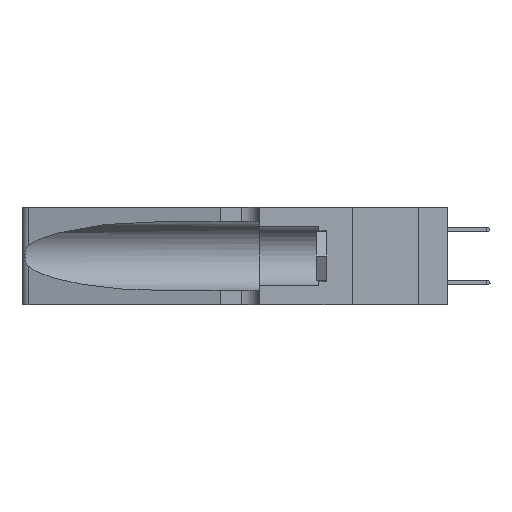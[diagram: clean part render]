
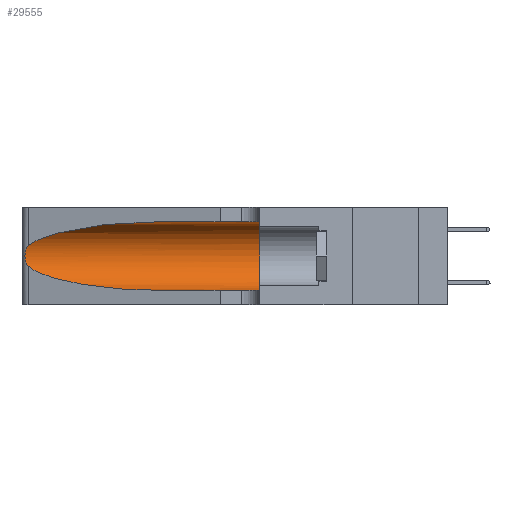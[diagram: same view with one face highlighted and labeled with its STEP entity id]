
A CAD part, left-side view. The second image highlights one B-rep face of the part: STEP entity #29555.
In plain terms, the highlighted cylindrical face has radius 3.308 mm (diameter 6.617 mm), a partial arc.
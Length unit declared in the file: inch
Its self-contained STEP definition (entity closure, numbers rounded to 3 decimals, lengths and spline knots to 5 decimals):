
#559 = CARTESIAN_POINT ( 'NONE',  ( 0.25787, 1.23484, 0.2124 ) ) ;
#2589 = CARTESIAN_POINT ( 'NONE',  ( 0.1305, 1.61858, 0.31525 ) ) ;
#2874 = ORIENTED_EDGE ( 'NONE', *, *, #18999, .T. ) ;
#3342 = CARTESIAN_POINT ( 'NONE',  ( 0.25856, 1.23593, 0.16098 ) ) ;
#3909 = CARTESIAN_POINT ( 'NONE',  ( 0.2373, 1.15595, 0.08982 ) ) ;
#4767 = ORIENTED_EDGE ( 'NONE', *, *, #8460, .T. ) ;
#4865 = DIRECTION ( 'NONE',  ( 0., 1., 0. ) ) ;
#4882 =( BOUNDED_CURVE ( )  B_SPLINE_CURVE ( 3, ( #11950, #3909, #14658, #31008 ),
 .UNSPECIFIED., .F., .F. ) 
 B_SPLINE_CURVE_WITH_KNOTS ( ( 4, 4 ),
 ( 3.44316, 4.71239 ),
 .UNSPECIFIED. ) 
 CURVE ( )  GEOMETRIC_REPRESENTATION_ITEM ( )  RATIONAL_B_SPLINE_CURVE ( ( 1., 0.87, 0.87, 1. ) ) 
 REPRESENTATION_ITEM ( '' )  );
#6047 = CARTESIAN_POINT ( 'NONE',  ( 0.25555, 1.22993, 0.14849 ) ) ;
#6652 = CARTESIAN_POINT ( 'NONE',  ( 0.1305, 1.61858, 0.185 ) ) ;
#6842 = CARTESIAN_POINT ( 'NONE',  ( 0.1305, 0.35, 0.31525 ) ) ;
#7187 = CARTESIAN_POINT ( 'NONE',  ( 0.1305, 0.72297, 0.31525 ) ) ;
#7802 = CARTESIAN_POINT ( 'NONE',  ( 0.1305, 0.72297, 0.31525 ) ) ;
#8460 = EDGE_CURVE ( 'NONE', #31767, #15767, #31958, .T. ) ;
#8649 = CARTESIAN_POINT ( 'NONE',  ( 0.26075, 1.23896, 0.19203 ) ) ;
#10161 = CARTESIAN_POINT ( 'NONE',  ( 0.18966, 0.96281, 0.31525 ) ) ;
#11276 = CARTESIAN_POINT ( 'NONE',  ( 0.25555, 1.22994, 0.2215 ) ) ;
#11371 = ORIENTED_EDGE ( 'NONE', *, *, #24735, .F. ) ;
#11396 = CARTESIAN_POINT ( 'NONE',  ( 0.26075, 1.23896, 0.178 ) ) ;
#11507 = CARTESIAN_POINT ( 'NONE',  ( 0.25487, 1.22718, 0.14631 ) ) ;
#11719 = LINE ( 'NONE', #24956, #23043 ) ;
#11950 = CARTESIAN_POINT ( 'NONE',  ( 0.25487, 1.22718, 0.14631 ) ) ;
#12204 = CARTESIAN_POINT ( 'NONE',  ( 0.25487, 1.22718, 0.14631 ) ) ;
#14658 = CARTESIAN_POINT ( 'NONE',  ( 0.18966, 0.96281, 0.05475 ) ) ;
#15136 = EDGE_CURVE ( 'NONE', #31767, #25947, #27100, .T. ) ;
#15450 = CARTESIAN_POINT ( 'NONE',  ( 0.2373, 1.15595, 0.28018 ) ) ;
#15749 = EDGE_CURVE ( 'NONE', #26336, #24824, #4882, .T. ) ;
#15767 = VERTEX_POINT ( 'NONE', #28085 ) ;
#16781 = CARTESIAN_POINT ( 'NONE',  ( 0.25789, 1.23486, 0.15765 ) ) ;
#17059 = CIRCLE ( 'NONE', #29937, 0.13025 ) ;
#18683 = FACE_OUTER_BOUND ( 'NONE', #33144, .T. ) ;
#18999 = EDGE_CURVE ( 'NONE', #15767, #26336, #33882, .T. ) ;
#19575 = DIRECTION ( 'NONE',  ( 0., -1., 0. ) ) ;
#20334 = CYLINDRICAL_SURFACE ( 'NONE', #22836, 0.13025 ) ;
#20994 = CARTESIAN_POINT ( 'NONE',  ( 0.1305, 0.35, 0.185 ) ) ;
#21076 = DIRECTION ( 'NONE',  ( 0., -1., 0. ) ) ;
#21408 = CARTESIAN_POINT ( 'NONE',  ( 0.1305, 0.72297, 0.05475 ) ) ;
#22061 = CARTESIAN_POINT ( 'NONE',  ( 0.25854, 1.2359, 0.20912 ) ) ;
#22167 = CARTESIAN_POINT ( 'NONE',  ( 0.25639, 1.23186, 0.15144 ) ) ;
#22613 = CARTESIAN_POINT ( 'NONE',  ( 0.1305, 0.35, 0.05475 ) ) ;
#22836 = AXIS2_PLACEMENT_3D ( 'NONE', #6652, #24653, #30121 ) ;
#23043 = VECTOR ( 'NONE', #19575, 39.37008 ) ;
#23219 = ORIENTED_EDGE ( 'NONE', *, *, #15749, .T. ) ;
#23647 = EDGE_CURVE ( 'NONE', #24824, #34590, #11719, .T. ) ;
#24653 = DIRECTION ( 'NONE',  ( 0., -1., 0. ) ) ;
#24735 = EDGE_CURVE ( 'NONE', #25947, #34590, #17059, .T. ) ;
#24753 = CARTESIAN_POINT ( 'NONE',  ( 0.26018, 1.23835, 0.19895 ) ) ;
#24824 = VERTEX_POINT ( 'NONE', #21408 ) ;
#24956 = CARTESIAN_POINT ( 'NONE',  ( 0.1305, 1.61858, 0.05475 ) ) ;
#25374 = ORIENTED_EDGE ( 'NONE', *, *, #15136, .F. ) ;
#25947 = VERTEX_POINT ( 'NONE', #6842 ) ;
#26336 = VERTEX_POINT ( 'NONE', #12204 ) ;
#27100 = LINE ( 'NONE', #2589, #29609 ) ;
#27318 = CARTESIAN_POINT ( 'NONE',  ( 0.25487, 1.22718, 0.22369 ) ) ;
#28085 = CARTESIAN_POINT ( 'NONE',  ( 0.25487, 1.22718, 0.22369 ) ) ;
#28301 = ORIENTED_EDGE ( 'NONE', *, *, #23647, .T. ) ;
#29555 = ADVANCED_FACE ( 'NONE', ( #18683 ), #20334, .F. ) ;
#29609 = VECTOR ( 'NONE', #21076, 39.37008 ) ;
#29937 = AXIS2_PLACEMENT_3D ( 'NONE', #20994, #4865, #31373 ) ;
#30121 = DIRECTION ( 'NONE',  ( 0., 0., -1. ) ) ;
#31008 = CARTESIAN_POINT ( 'NONE',  ( 0.1305, 0.72297, 0.05475 ) ) ;
#31373 = DIRECTION ( 'NONE',  ( 0., 0., 1. ) ) ;
#31767 = VERTEX_POINT ( 'NONE', #7802 ) ;
#31958 =( BOUNDED_CURVE ( )  B_SPLINE_CURVE ( 3, ( #7187, #10161, #15450, #34002 ),
 .UNSPECIFIED., .F., .F. ) 
 B_SPLINE_CURVE_WITH_KNOTS ( ( 4, 4 ),
 ( 1.5708, 2.84003 ),
 .UNSPECIFIED. ) 
 CURVE ( )  GEOMETRIC_REPRESENTATION_ITEM ( )  RATIONAL_B_SPLINE_CURVE ( ( 1., 0.87, 0.87, 1. ) ) 
 REPRESENTATION_ITEM ( '' )  );
#32655 = CARTESIAN_POINT ( 'NONE',  ( 0.25639, 1.23184, 0.21858 ) ) ;
#32771 = CARTESIAN_POINT ( 'NONE',  ( 0.26017, 1.23833, 0.17102 ) ) ;
#33144 = EDGE_LOOP ( 'NONE', ( #4767, #2874, #23219, #28301, #11371, #25374 ) ) ;
#33882 = B_SPLINE_CURVE_WITH_KNOTS ( 'NONE', 3,
 ( #27318, #11276, #32655, #559, #22061, #24753, #8649, #11396, #32771, #3342, #16781, #22167, #6047, #11507 ),
 .UNSPECIFIED., .F., .F.,
 ( 4, 2, 2, 2, 2, 2, 4 ),
 ( 0., 0.00027, 0.00053, 0.00107, 0.0016, 0.00187, 0.00214 ),
 .UNSPECIFIED. ) ;
#34002 = CARTESIAN_POINT ( 'NONE',  ( 0.25487, 1.22718, 0.22369 ) ) ;
#34590 = VERTEX_POINT ( 'NONE', #22613 ) ;
